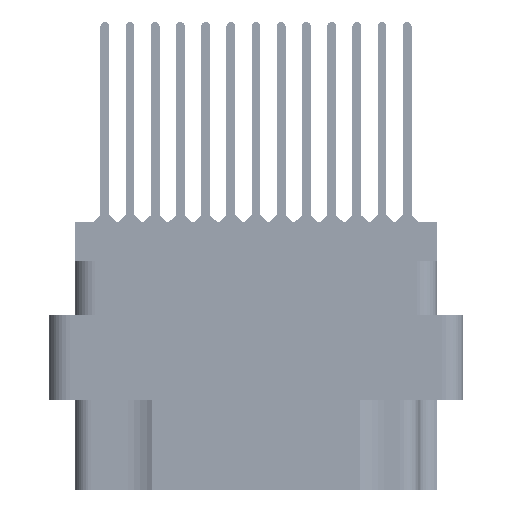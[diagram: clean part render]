
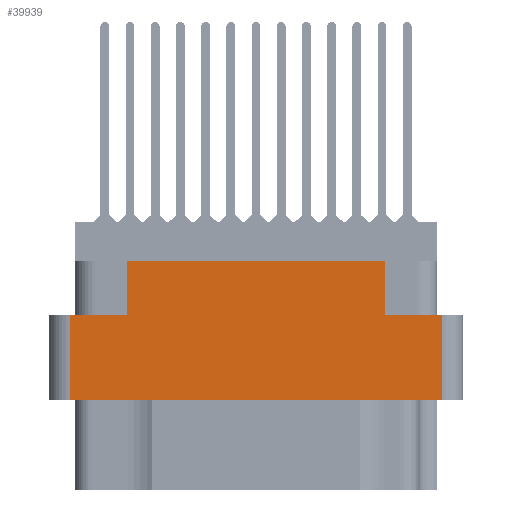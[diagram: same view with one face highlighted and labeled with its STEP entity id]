
A CAD part, left-side view. The second image highlights one B-rep face of the part: STEP entity #39939.
In plain terms, the highlighted planar face has unit normal (-1, 0, 0).
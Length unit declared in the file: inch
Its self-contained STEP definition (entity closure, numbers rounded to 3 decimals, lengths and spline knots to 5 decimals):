
#587 = ORIENTED_EDGE ( 'NONE', *, *, #64719, .F. ) ;
#822 = VECTOR ( 'NONE', #14557, 39.37008 ) ;
#850 = ORIENTED_EDGE ( 'NONE', *, *, #48883, .T. ) ;
#1000 = LINE ( 'NONE', #2486, #33328 ) ;
#1086 = ORIENTED_EDGE ( 'NONE', *, *, #30590, .F. ) ;
#1295 = EDGE_CURVE ( 'NONE', #17829, #30019, #61709, .T. ) ;
#1522 = EDGE_LOOP ( 'NONE', ( #587, #71474, #73766, #52041, #37520, #850, #45826, #1086 ) ) ;
#1998 = EDGE_CURVE ( 'NONE', #65715, #65966, #53520, .T. ) ;
#2486 = CARTESIAN_POINT ( 'NONE',  ( -1.359, 0., -0.529 ) ) ;
#6538 = DIRECTION ( 'NONE',  ( -1., 0., 0. ) ) ;
#6651 = LINE ( 'NONE', #66545, #65759 ) ;
#6759 = CARTESIAN_POINT ( 'NONE',  ( -1.359, 0.3825, -0.117 ) ) ;
#7153 = CARTESIAN_POINT ( 'NONE',  ( -1.359, -0.555, -0.529 ) ) ;
#8937 = VECTOR ( 'NONE', #67725, 39.37008 ) ;
#10819 = DIRECTION ( 'NONE',  ( 0., 0., 1. ) ) ;
#14307 = CARTESIAN_POINT ( 'NONE',  ( -1.359, -0.555, -0.798 ) ) ;
#14557 = DIRECTION ( 'NONE',  ( 0., 0., 1. ) ) ;
#17829 = VERTEX_POINT ( 'NONE', #7153 ) ;
#18043 = PLANE ( 'NONE',  #72424 ) ;
#19128 = VERTEX_POINT ( 'NONE', #59539 ) ;
#19679 = EDGE_CURVE ( 'NONE', #17829, #56368, #1000, .T. ) ;
#19848 = DIRECTION ( 'NONE',  ( 0., 0., -1. ) ) ;
#20483 = CARTESIAN_POINT ( 'NONE',  ( -1.359, 0.3825, -0.277 ) ) ;
#20755 = CARTESIAN_POINT ( 'NONE',  ( -1.359, -0.3825, -0.117 ) ) ;
#20850 = CARTESIAN_POINT ( 'NONE',  ( -1.359, 0.555, -0.798 ) ) ;
#22511 = CARTESIAN_POINT ( 'NONE',  ( -1.359, 0., -0.277 ) ) ;
#23082 = VECTOR ( 'NONE', #10819, 39.37008 ) ;
#24812 = DIRECTION ( 'NONE',  ( 0., 1., 0. ) ) ;
#25582 = FACE_OUTER_BOUND ( 'NONE', #1522, .T. ) ;
#26603 = DIRECTION ( 'NONE',  ( 0., -1., 0. ) ) ;
#27618 = VECTOR ( 'NONE', #50333, 39.37008 ) ;
#28140 = CARTESIAN_POINT ( 'NONE',  ( -1.359, 0.617, -0.117 ) ) ;
#28372 = VECTOR ( 'NONE', #19848, 39.37008 ) ;
#30019 = VERTEX_POINT ( 'NONE', #39921 ) ;
#30440 = VERTEX_POINT ( 'NONE', #20483 ) ;
#30590 = EDGE_CURVE ( 'NONE', #30440, #65715, #61805, .T. ) ;
#33328 = VECTOR ( 'NONE', #24812, 39.37008 ) ;
#35175 = CARTESIAN_POINT ( 'NONE',  ( -1.359, -0.617, -0.798 ) ) ;
#37520 = ORIENTED_EDGE ( 'NONE', *, *, #55606, .F. ) ;
#39822 = VECTOR ( 'NONE', #40614, 39.37008 ) ;
#39921 = CARTESIAN_POINT ( 'NONE',  ( -1.359, -0.555, -0.277 ) ) ;
#39939 = ADVANCED_FACE ( 'NONE', ( #25582 ), #18043, .T. ) ;
#40614 = DIRECTION ( 'NONE',  ( 0., -1., 0. ) ) ;
#43340 = EDGE_CURVE ( 'NONE', #45944, #56368, #43597, .T. ) ;
#43597 = LINE ( 'NONE', #20850, #28372 ) ;
#45826 = ORIENTED_EDGE ( 'NONE', *, *, #1998, .F. ) ;
#45944 = VERTEX_POINT ( 'NONE', #46025 ) ;
#46025 = CARTESIAN_POINT ( 'NONE',  ( -1.359, 0.555, -0.277 ) ) ;
#48883 = EDGE_CURVE ( 'NONE', #19128, #65966, #65112, .T. ) ;
#50333 = DIRECTION ( 'NONE',  ( 0., -1., 0. ) ) ;
#50613 = CARTESIAN_POINT ( 'NONE',  ( -1.359, -0.3825, -0.277 ) ) ;
#52041 = ORIENTED_EDGE ( 'NONE', *, *, #1295, .T. ) ;
#53520 = LINE ( 'NONE', #28140, #27618 ) ;
#55606 = EDGE_CURVE ( 'NONE', #19128, #30019, #59360, .T. ) ;
#56368 = VERTEX_POINT ( 'NONE', #70901 ) ;
#59360 = LINE ( 'NONE', #22511, #39822 ) ;
#59539 = CARTESIAN_POINT ( 'NONE',  ( -1.359, -0.3825, -0.277 ) ) ;
#61709 = LINE ( 'NONE', #14307, #822 ) ;
#61757 = CARTESIAN_POINT ( 'NONE',  ( -1.359, 0.3825, -0.277 ) ) ;
#61805 = LINE ( 'NONE', #61757, #8937 ) ;
#63108 = DIRECTION ( 'NONE',  ( 0., 0., 1. ) ) ;
#64719 = EDGE_CURVE ( 'NONE', #45944, #30440, #6651, .T. ) ;
#65112 = LINE ( 'NONE', #50613, #23082 ) ;
#65715 = VERTEX_POINT ( 'NONE', #6759 ) ;
#65759 = VECTOR ( 'NONE', #26603, 39.37008 ) ;
#65966 = VERTEX_POINT ( 'NONE', #20755 ) ;
#66545 = CARTESIAN_POINT ( 'NONE',  ( -1.359, 0., -0.277 ) ) ;
#67725 = DIRECTION ( 'NONE',  ( 0., 0., 1. ) ) ;
#70901 = CARTESIAN_POINT ( 'NONE',  ( -1.359, 0.555, -0.529 ) ) ;
#71474 = ORIENTED_EDGE ( 'NONE', *, *, #43340, .T. ) ;
#72424 = AXIS2_PLACEMENT_3D ( 'NONE', #35175, #6538, #63108 ) ;
#73766 = ORIENTED_EDGE ( 'NONE', *, *, #19679, .F. ) ;
